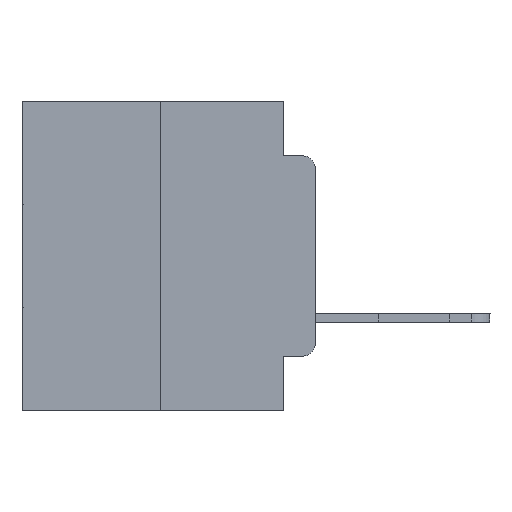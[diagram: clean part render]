
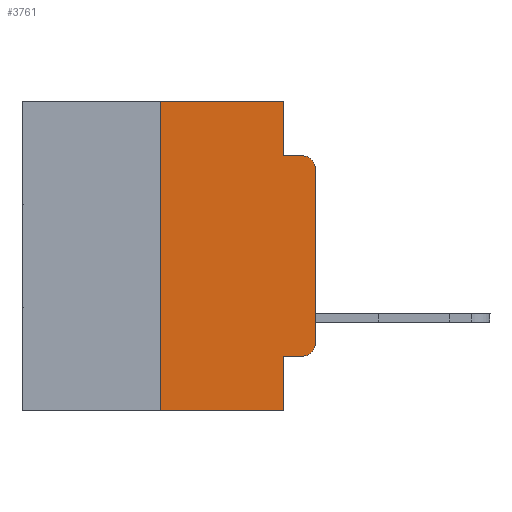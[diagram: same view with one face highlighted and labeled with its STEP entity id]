
A CAD part, left-side view. The second image highlights one B-rep face of the part: STEP entity #3761.
In plain terms, the highlighted planar face has unit normal (-1, 0, 0).
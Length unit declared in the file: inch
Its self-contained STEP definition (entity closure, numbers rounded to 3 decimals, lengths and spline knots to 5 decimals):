
#227 = AXIS2_PLACEMENT_3D ( 'NONE', #21699, #21547, #21727 ) ;
#246 = VERTEX_POINT ( 'NONE', #8210 ) ;
#1647 = EDGE_CURVE ( 'NONE', #2607, #23612, #13671, .T. ) ;
#1674 = DIRECTION ( 'NONE',  ( 0., 0., 1. ) ) ;
#1836 = LINE ( 'NONE', #22973, #26333 ) ;
#2071 = ORIENTED_EDGE ( 'NONE', *, *, #27054, .F. ) ;
#2607 = VERTEX_POINT ( 'NONE', #15635 ) ;
#2660 = CARTESIAN_POINT ( 'NONE',  ( 0., 0.473, -0.5 ) ) ;
#2759 = ORIENTED_EDGE ( 'NONE', *, *, #8811, .T. ) ;
#2833 = VERTEX_POINT ( 'NONE', #4967 ) ;
#2960 = DIRECTION ( 'NONE',  ( 0., 0., -1. ) ) ;
#3689 = LINE ( 'NONE', #20738, #7956 ) ;
#3761 = ADVANCED_FACE ( 'NONE', ( #18246 ), #19536, .F. ) ;
#3858 = DIRECTION ( 'NONE',  ( 0., 0., -1. ) ) ;
#4102 = DIRECTION ( 'NONE',  ( 0., 0., -1. ) ) ;
#4435 = CARTESIAN_POINT ( 'NONE',  ( 0., 0.051, -0.4115 ) ) ;
#4967 = CARTESIAN_POINT ( 'NONE',  ( 0., 0.051, -0.0885 ) ) ;
#5970 = DIRECTION ( 'NONE',  ( 0., 0., -1. ) ) ;
#6737 = ORIENTED_EDGE ( 'NONE', *, *, #20393, .F. ) ;
#7047 = EDGE_CURVE ( 'NONE', #13076, #2607, #24157, .T. ) ;
#7416 = VECTOR ( 'NONE', #21518, 39.37008 ) ;
#7956 = VECTOR ( 'NONE', #4102, 39.37008 ) ;
#8210 = CARTESIAN_POINT ( 'NONE',  ( 0., 0.02, -0.4115 ) ) ;
#8296 = VERTEX_POINT ( 'NONE', #12480 ) ;
#8334 = EDGE_LOOP ( 'NONE', ( #15856, #13278, #6737, #11203, #11607, #2071, #19139, #20720, #26301, #2759 ) ) ;
#8687 = LINE ( 'NONE', #21482, #15985 ) ;
#8811 = EDGE_CURVE ( 'NONE', #246, #13076, #27415, .T. ) ;
#9524 = LINE ( 'NONE', #4435, #19241 ) ;
#9874 = CARTESIAN_POINT ( 'NONE',  ( 0., 0.051, -0.4115 ) ) ;
#10416 = DIRECTION ( 'NONE',  ( 0., -1., 0. ) ) ;
#11023 = VERTEX_POINT ( 'NONE', #17927 ) ;
#11203 = ORIENTED_EDGE ( 'NONE', *, *, #12474, .F. ) ;
#11607 = ORIENTED_EDGE ( 'NONE', *, *, #21164, .F. ) ;
#12474 = EDGE_CURVE ( 'NONE', #11023, #2833, #3689, .T. ) ;
#12480 = CARTESIAN_POINT ( 'NONE',  ( 0., 0.25, 0. ) ) ;
#12700 = CARTESIAN_POINT ( 'NONE',  ( 0., 0., -0.3915 ) ) ;
#12877 = VERTEX_POINT ( 'NONE', #9874 ) ;
#13076 = VERTEX_POINT ( 'NONE', #12700 ) ;
#13202 = VERTEX_POINT ( 'NONE', #23990 ) ;
#13278 = ORIENTED_EDGE ( 'NONE', *, *, #1647, .T. ) ;
#13671 = CIRCLE ( 'NONE', #18826, 0.02 ) ;
#13730 = EDGE_CURVE ( 'NONE', #12877, #246, #9524, .T. ) ;
#14080 = AXIS2_PLACEMENT_3D ( 'NONE', #20682, #27235, #5970 ) ;
#14906 = CARTESIAN_POINT ( 'NONE',  ( 0., 0.051, -0.5 ) ) ;
#15635 = CARTESIAN_POINT ( 'NONE',  ( 0., 0., -0.1085 ) ) ;
#15856 = ORIENTED_EDGE ( 'NONE', *, *, #7047, .T. ) ;
#15985 = VECTOR ( 'NONE', #22221, 39.37008 ) ;
#16192 = LINE ( 'NONE', #2660, #20549 ) ;
#16367 = CARTESIAN_POINT ( 'NONE',  ( 0., 0.02, -0.1085 ) ) ;
#17203 = CARTESIAN_POINT ( 'NONE',  ( 0., 0.051, -0.0885 ) ) ;
#17927 = CARTESIAN_POINT ( 'NONE',  ( 0., 0.051, 0. ) ) ;
#18140 = VERTEX_POINT ( 'NONE', #14906 ) ;
#18246 = FACE_OUTER_BOUND ( 'NONE', #8334, .T. ) ;
#18826 = AXIS2_PLACEMENT_3D ( 'NONE', #16367, #20692, #3858 ) ;
#19139 = ORIENTED_EDGE ( 'NONE', *, *, #25826, .T. ) ;
#19241 = VECTOR ( 'NONE', #10416, 39.37008 ) ;
#19536 = PLANE ( 'NONE',  #227 ) ;
#19900 = CARTESIAN_POINT ( 'NONE',  ( 0., 0.02, -0.0885 ) ) ;
#20393 = EDGE_CURVE ( 'NONE', #2833, #23612, #25112, .T. ) ;
#20549 = VECTOR ( 'NONE', #23699, 39.37008 ) ;
#20552 = DIRECTION ( 'NONE',  ( 0., 0., 1. ) ) ;
#20682 = CARTESIAN_POINT ( 'NONE',  ( 0., 0.02, -0.3915 ) ) ;
#20692 = DIRECTION ( 'NONE',  ( -1., 0., 0. ) ) ;
#20720 = ORIENTED_EDGE ( 'NONE', *, *, #27516, .F. ) ;
#20738 = CARTESIAN_POINT ( 'NONE',  ( 0., 0.051, 0. ) ) ;
#21164 = EDGE_CURVE ( 'NONE', #8296, #11023, #8687, .T. ) ;
#21482 = CARTESIAN_POINT ( 'NONE',  ( 0., 0.473, 0. ) ) ;
#21518 = DIRECTION ( 'NONE',  ( 0., -1., 0. ) ) ;
#21547 = DIRECTION ( 'NONE',  ( 1., 0., 0. ) ) ;
#21699 = CARTESIAN_POINT ( 'NONE',  ( 0., 0.473, 0. ) ) ;
#21727 = DIRECTION ( 'NONE',  ( 0., 0., -1. ) ) ;
#22221 = DIRECTION ( 'NONE',  ( 0., -1., 0. ) ) ;
#22973 = CARTESIAN_POINT ( 'NONE',  ( 0., 0.25, 0. ) ) ;
#23612 = VERTEX_POINT ( 'NONE', #19900 ) ;
#23699 = DIRECTION ( 'NONE',  ( 0., -1., 0. ) ) ;
#23990 = CARTESIAN_POINT ( 'NONE',  ( 0., 0.25, -0.5 ) ) ;
#24157 = LINE ( 'NONE', #26917, #25142 ) ;
#25112 = LINE ( 'NONE', #17203, #7416 ) ;
#25142 = VECTOR ( 'NONE', #20552, 39.37008 ) ;
#25332 = LINE ( 'NONE', #26342, #26031 ) ;
#25826 = EDGE_CURVE ( 'NONE', #13202, #18140, #16192, .T. ) ;
#26031 = VECTOR ( 'NONE', #2960, 39.37008 ) ;
#26301 = ORIENTED_EDGE ( 'NONE', *, *, #13730, .T. ) ;
#26333 = VECTOR ( 'NONE', #1674, 39.37008 ) ;
#26342 = CARTESIAN_POINT ( 'NONE',  ( 0., 0.051, 0. ) ) ;
#26917 = CARTESIAN_POINT ( 'NONE',  ( 0., 0., 0. ) ) ;
#27054 = EDGE_CURVE ( 'NONE', #13202, #8296, #1836, .T. ) ;
#27235 = DIRECTION ( 'NONE',  ( -1., 0., 0. ) ) ;
#27415 = CIRCLE ( 'NONE', #14080, 0.02 ) ;
#27516 = EDGE_CURVE ( 'NONE', #12877, #18140, #25332, .T. ) ;
